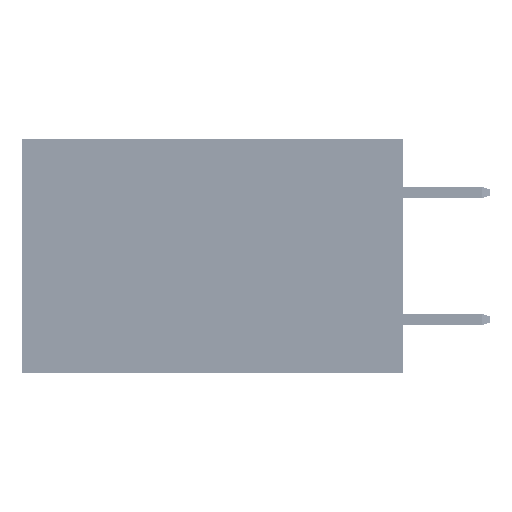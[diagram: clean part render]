
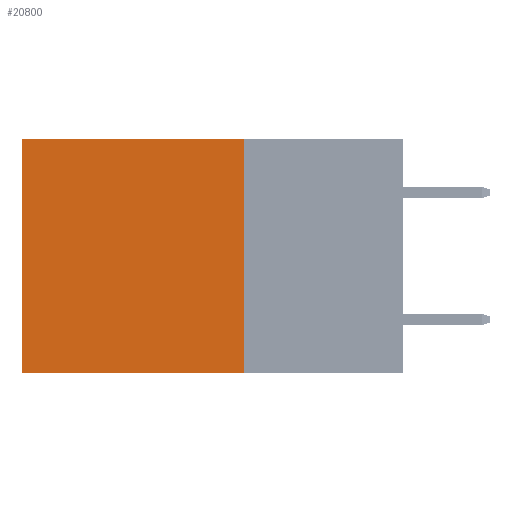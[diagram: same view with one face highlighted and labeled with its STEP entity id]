
A CAD part, left-side view. The second image highlights one B-rep face of the part: STEP entity #20800.
In plain terms, the highlighted planar face has unit normal (-1, 0, 0).
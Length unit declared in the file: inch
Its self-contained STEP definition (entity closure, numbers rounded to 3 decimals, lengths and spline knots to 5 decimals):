
#930 = CARTESIAN_POINT ( 'NONE',  ( 0.2875, 0.25, 0. ) ) ;
#1188 = VECTOR ( 'NONE', #37788, 39.37008 ) ;
#1809 = CARTESIAN_POINT ( 'NONE',  ( 0.2875, 0.25, -0.37 ) ) ;
#2445 = LINE ( 'NONE', #17794, #1188 ) ;
#2522 = VECTOR ( 'NONE', #42767, 39.37008 ) ;
#3544 = EDGE_LOOP ( 'NONE', ( #25049, #10856, #21496, #23795 ) ) ;
#7227 = VERTEX_POINT ( 'NONE', #1809 ) ;
#7973 = EDGE_CURVE ( 'NONE', #18068, #7227, #2445, .T. ) ;
#9948 = CARTESIAN_POINT ( 'NONE',  ( 0.2875, 0.25, -0.37 ) ) ;
#10428 = VERTEX_POINT ( 'NONE', #43718 ) ;
#10856 = ORIENTED_EDGE ( 'NONE', *, *, #12486, .F. ) ;
#11341 = LINE ( 'NONE', #19932, #2522 ) ;
#12436 = CARTESIAN_POINT ( 'NONE',  ( 0.2875, 0.6, 0. ) ) ;
#12486 = EDGE_CURVE ( 'NONE', #7227, #10428, #40574, .T. ) ;
#12936 = LINE ( 'NONE', #12436, #27758 ) ;
#17007 = DIRECTION ( 'NONE',  ( 0., 1., 0. ) ) ;
#17794 = CARTESIAN_POINT ( 'NONE',  ( 0.2875, 0.25, 0. ) ) ;
#18068 = VERTEX_POINT ( 'NONE', #930 ) ;
#18694 = VERTEX_POINT ( 'NONE', #33223 ) ;
#19932 = CARTESIAN_POINT ( 'NONE',  ( 0.2875, 0.25, 0. ) ) ;
#20800 = ADVANCED_FACE ( 'NONE', ( #28545 ), #47819, .F. ) ;
#21496 = ORIENTED_EDGE ( 'NONE', *, *, #7973, .F. ) ;
#23795 = ORIENTED_EDGE ( 'NONE', *, *, #45786, .T. ) ;
#24463 = DIRECTION ( 'NONE',  ( 1., 0., 0. ) ) ;
#25049 = ORIENTED_EDGE ( 'NONE', *, *, #35956, .T. ) ;
#27758 = VECTOR ( 'NONE', #43867, 39.37008 ) ;
#28545 = FACE_OUTER_BOUND ( 'NONE', #3544, .T. ) ;
#29045 = DIRECTION ( 'NONE',  ( 0., 0., -1. ) ) ;
#33223 = CARTESIAN_POINT ( 'NONE',  ( 0.2875, 0.6, 0. ) ) ;
#35956 = EDGE_CURVE ( 'NONE', #18694, #10428, #12936, .T. ) ;
#36061 = VECTOR ( 'NONE', #17007, 39.37008 ) ;
#36163 = CARTESIAN_POINT ( 'NONE',  ( 0.2875, 0.25, 0. ) ) ;
#37788 = DIRECTION ( 'NONE',  ( 0., 0., -1. ) ) ;
#40574 = LINE ( 'NONE', #9948, #36061 ) ;
#41324 = AXIS2_PLACEMENT_3D ( 'NONE', #36163, #24463, #29045 ) ;
#42767 = DIRECTION ( 'NONE',  ( 0., 1., 0. ) ) ;
#43718 = CARTESIAN_POINT ( 'NONE',  ( 0.2875, 0.6, -0.37 ) ) ;
#43867 = DIRECTION ( 'NONE',  ( 0., 0., -1. ) ) ;
#45786 = EDGE_CURVE ( 'NONE', #18068, #18694, #11341, .T. ) ;
#47819 = PLANE ( 'NONE',  #41324 ) ;
